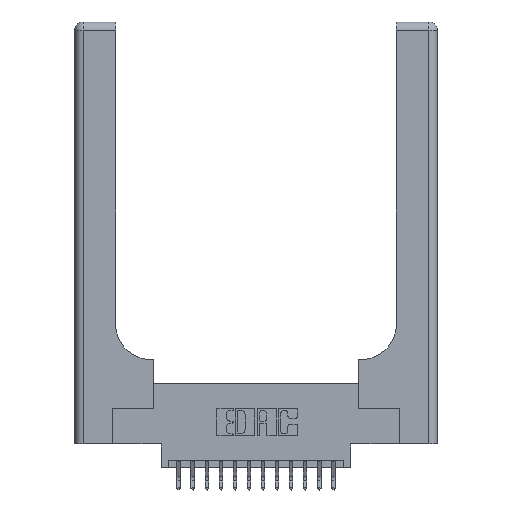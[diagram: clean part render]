
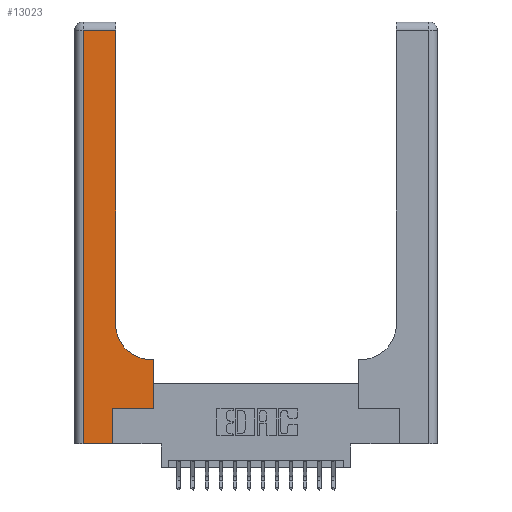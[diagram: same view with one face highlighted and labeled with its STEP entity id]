
A CAD part, top view. The second image highlights one B-rep face of the part: STEP entity #13023.
In plain terms, the highlighted planar face has unit normal (0, 0, 1).
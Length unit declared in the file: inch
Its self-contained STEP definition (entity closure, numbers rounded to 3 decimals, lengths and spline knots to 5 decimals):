
#133 = CIRCLE ( 'NONE', #8551, 0.25 ) ;
#924 = PLANE ( 'NONE',  #1505 ) ;
#1131 = EDGE_CURVE ( 'NONE', #12037, #15858, #11486, .T. ) ;
#1226 = ORIENTED_EDGE ( 'NONE', *, *, #8321, .T. ) ;
#1301 = ORIENTED_EDGE ( 'NONE', *, *, #1131, .T. ) ;
#1505 = AXIS2_PLACEMENT_3D ( 'NONE', #9897, #11257, #8413 ) ;
#1576 = LINE ( 'NONE', #4154, #16748 ) ;
#1702 = DIRECTION ( 'NONE',  ( -1., 0., 0. ) ) ;
#2062 = EDGE_CURVE ( 'NONE', #7625, #5169, #8687, .T. ) ;
#2465 = LINE ( 'NONE', #4991, #11212 ) ;
#2584 = VERTEX_POINT ( 'NONE', #13336 ) ;
#2615 = CARTESIAN_POINT ( 'NONE',  ( 0., 2.94, 0.37 ) ) ;
#2644 = CARTESIAN_POINT ( 'NONE',  ( 0.5415, 0.85, 0.37 ) ) ;
#2796 = DIRECTION ( 'NONE',  ( 1., 0., 0. ) ) ;
#2892 = EDGE_CURVE ( 'NONE', #18065, #9921, #2465, .T. ) ;
#3863 = EDGE_CURVE ( 'NONE', #5169, #18065, #18477, .T. ) ;
#4154 = CARTESIAN_POINT ( 'NONE',  ( 0.269, 0.25, 0.37 ) ) ;
#4418 = ORIENTED_EDGE ( 'NONE', *, *, #2062, .T. ) ;
#4991 = CARTESIAN_POINT ( 'NONE',  ( 0.06, 3., 0.37 ) ) ;
#5169 = VERTEX_POINT ( 'NONE', #6036 ) ;
#5262 = VECTOR ( 'NONE', #6452, 39.37008 ) ;
#5655 = VERTEX_POINT ( 'NONE', #5931 ) ;
#5809 = EDGE_LOOP ( 'NONE', ( #4418, #12761, #14330, #10757, #1301, #1226, #11621, #10305, #14250 ) ) ;
#5863 = CARTESIAN_POINT ( 'NONE',  ( 0.2915, 3., 0.37 ) ) ;
#5931 = CARTESIAN_POINT ( 'NONE',  ( 0.5585, 0.6, 0.37 ) ) ;
#6036 = CARTESIAN_POINT ( 'NONE',  ( 0.2915, 2.94, 0.37 ) ) ;
#6452 = DIRECTION ( 'NONE',  ( 0., 1., 0. ) ) ;
#6597 = CARTESIAN_POINT ( 'NONE',  ( 0.269, 0.25, 0.37 ) ) ;
#7550 = VECTOR ( 'NONE', #1702, 39.37008 ) ;
#7625 = VERTEX_POINT ( 'NONE', #12677 ) ;
#7641 = CARTESIAN_POINT ( 'NONE',  ( 0., 0., 0.37 ) ) ;
#8321 = EDGE_CURVE ( 'NONE', #15858, #13643, #1576, .T. ) ;
#8332 = CARTESIAN_POINT ( 'NONE',  ( 0.5585, 0.25, 0.37 ) ) ;
#8413 = DIRECTION ( 'NONE',  ( -1., 0., 0. ) ) ;
#8551 = AXIS2_PLACEMENT_3D ( 'NONE', #2644, #12914, #14374 ) ;
#8687 = LINE ( 'NONE', #5863, #17584 ) ;
#8707 = VECTOR ( 'NONE', #11048, 39.37008 ) ;
#8750 = VECTOR ( 'NONE', #14929, 39.37008 ) ;
#9561 = FACE_OUTER_BOUND ( 'NONE', #5809, .T. ) ;
#9646 = LINE ( 'NONE', #18091, #5262 ) ;
#9897 = CARTESIAN_POINT ( 'NONE',  ( 0., 3., 0.37 ) ) ;
#9921 = VERTEX_POINT ( 'NONE', #11923 ) ;
#10305 = ORIENTED_EDGE ( 'NONE', *, *, #17108, .T. ) ;
#10426 = CARTESIAN_POINT ( 'NONE',  ( 0.269, 0., 0.37 ) ) ;
#10757 = ORIENTED_EDGE ( 'NONE', *, *, #15300, .T. ) ;
#10801 = CARTESIAN_POINT ( 'NONE',  ( 0.2915, 0.6, 0.37 ) ) ;
#11048 = DIRECTION ( 'NONE',  ( 0., 1., 0. ) ) ;
#11212 = VECTOR ( 'NONE', #16696, 39.37008 ) ;
#11257 = DIRECTION ( 'NONE',  ( 0., 0., -1. ) ) ;
#11486 = LINE ( 'NONE', #13971, #8707 ) ;
#11621 = ORIENTED_EDGE ( 'NONE', *, *, #16167, .T. ) ;
#11923 = CARTESIAN_POINT ( 'NONE',  ( 0.06, 0., 0.37 ) ) ;
#11982 = EDGE_CURVE ( 'NONE', #2584, #7625, #133, .T. ) ;
#12037 = VERTEX_POINT ( 'NONE', #10426 ) ;
#12677 = CARTESIAN_POINT ( 'NONE',  ( 0.2915, 0.85, 0.37 ) ) ;
#12761 = ORIENTED_EDGE ( 'NONE', *, *, #3863, .T. ) ;
#12914 = DIRECTION ( 'NONE',  ( 0., 0., -1. ) ) ;
#13023 = ADVANCED_FACE ( 'NONE', ( #9561 ), #924, .F. ) ;
#13336 = CARTESIAN_POINT ( 'NONE',  ( 0.5415, 0.6, 0.37 ) ) ;
#13643 = VERTEX_POINT ( 'NONE', #8332 ) ;
#13971 = CARTESIAN_POINT ( 'NONE',  ( 0.269, 0., 0.37 ) ) ;
#14030 = LINE ( 'NONE', #7641, #8750 ) ;
#14250 = ORIENTED_EDGE ( 'NONE', *, *, #11982, .T. ) ;
#14255 = CARTESIAN_POINT ( 'NONE',  ( 0.06, 2.94, 0.37 ) ) ;
#14330 = ORIENTED_EDGE ( 'NONE', *, *, #2892, .T. ) ;
#14374 = DIRECTION ( 'NONE',  ( 1., 0., 0. ) ) ;
#14929 = DIRECTION ( 'NONE',  ( 1., 0., 0. ) ) ;
#15300 = EDGE_CURVE ( 'NONE', #9921, #12037, #14030, .T. ) ;
#15858 = VERTEX_POINT ( 'NONE', #6597 ) ;
#16167 = EDGE_CURVE ( 'NONE', #13643, #5655, #9646, .T. ) ;
#16255 = LINE ( 'NONE', #10801, #7550 ) ;
#16696 = DIRECTION ( 'NONE',  ( 0., -1., 0. ) ) ;
#16748 = VECTOR ( 'NONE', #2796, 39.37008 ) ;
#17108 = EDGE_CURVE ( 'NONE', #5655, #2584, #16255, .T. ) ;
#17554 = VECTOR ( 'NONE', #18599, 39.37008 ) ;
#17564 = DIRECTION ( 'NONE',  ( 0., 1., 0. ) ) ;
#17584 = VECTOR ( 'NONE', #17564, 39.37008 ) ;
#18065 = VERTEX_POINT ( 'NONE', #14255 ) ;
#18091 = CARTESIAN_POINT ( 'NONE',  ( 0.5585, 0.25, 0.37 ) ) ;
#18477 = LINE ( 'NONE', #2615, #17554 ) ;
#18599 = DIRECTION ( 'NONE',  ( -1., 0., 0. ) ) ;
